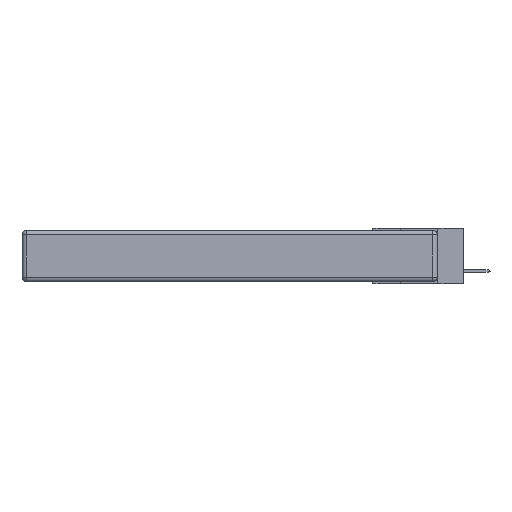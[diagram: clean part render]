
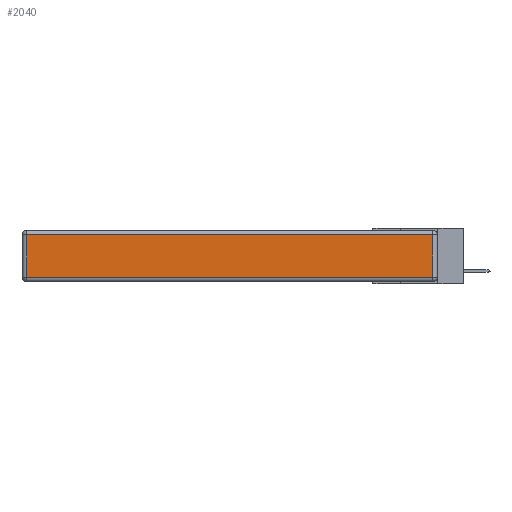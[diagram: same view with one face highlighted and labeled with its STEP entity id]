
A CAD part, left-side view. The second image highlights one B-rep face of the part: STEP entity #2040.
In plain terms, the highlighted planar face has unit normal (-1, 0, 0).
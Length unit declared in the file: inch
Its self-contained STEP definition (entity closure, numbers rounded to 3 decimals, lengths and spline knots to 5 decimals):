
#252 = VECTOR ( 'NONE', #1805, 39.37008 ) ;
#397 = CARTESIAN_POINT ( 'NONE',  ( 0., 2.72, -0.313 ) ) ;
#528 = CARTESIAN_POINT ( 'NONE',  ( 0., 0.03, -0.343 ) ) ;
#615 = EDGE_CURVE ( 'NONE', #8785, #6904, #5370, .T. ) ;
#1092 = ORIENTED_EDGE ( 'NONE', *, *, #615, .T. ) ;
#1435 = VECTOR ( 'NONE', #5784, 39.37008 ) ;
#1805 = DIRECTION ( 'NONE',  ( 0., 0., 1. ) ) ;
#2040 = ADVANCED_FACE ( 'NONE', ( #12250 ), #4690, .T. ) ;
#2450 = VERTEX_POINT ( 'NONE', #397 ) ;
#3896 = VECTOR ( 'NONE', #12464, 39.37008 ) ;
#4378 = EDGE_LOOP ( 'NONE', ( #11675, #1092, #7828, #9726 ) ) ;
#4491 = EDGE_CURVE ( 'NONE', #6904, #4691, #7237, .T. ) ;
#4690 = PLANE ( 'NONE',  #10611 ) ;
#4691 = VERTEX_POINT ( 'NONE', #9152 ) ;
#4716 = CARTESIAN_POINT ( 'NONE',  ( 0., 0.03, -0.313 ) ) ;
#4989 = LINE ( 'NONE', #13332, #1435 ) ;
#5370 = LINE ( 'NONE', #528, #252 ) ;
#5624 = CARTESIAN_POINT ( 'NONE',  ( 0., 0.03, -0.03 ) ) ;
#5784 = DIRECTION ( 'NONE',  ( 0., -1., 0. ) ) ;
#5982 = CARTESIAN_POINT ( 'NONE',  ( 0., 0., -0.343 ) ) ;
#6904 = VERTEX_POINT ( 'NONE', #5624 ) ;
#7237 = LINE ( 'NONE', #16169, #3896 ) ;
#7244 = DIRECTION ( 'NONE',  ( -1., 0., 0. ) ) ;
#7828 = ORIENTED_EDGE ( 'NONE', *, *, #4491, .T. ) ;
#8142 = EDGE_CURVE ( 'NONE', #2450, #8785, #4989, .T. ) ;
#8517 = DIRECTION ( 'NONE',  ( 0., 0., 1. ) ) ;
#8785 = VERTEX_POINT ( 'NONE', #4716 ) ;
#9152 = CARTESIAN_POINT ( 'NONE',  ( 0., 2.72, -0.03 ) ) ;
#9726 = ORIENTED_EDGE ( 'NONE', *, *, #14651, .T. ) ;
#10611 = AXIS2_PLACEMENT_3D ( 'NONE', #5982, #7244, #8517 ) ;
#11675 = ORIENTED_EDGE ( 'NONE', *, *, #8142, .T. ) ;
#12235 = VECTOR ( 'NONE', #15403, 39.37008 ) ;
#12250 = FACE_OUTER_BOUND ( 'NONE', #4378, .T. ) ;
#12464 = DIRECTION ( 'NONE',  ( 0., 1., 0. ) ) ;
#13018 = LINE ( 'NONE', #14205, #12235 ) ;
#13332 = CARTESIAN_POINT ( 'NONE',  ( 0., 0., -0.313 ) ) ;
#14205 = CARTESIAN_POINT ( 'NONE',  ( 0., 2.72, -0.343 ) ) ;
#14651 = EDGE_CURVE ( 'NONE', #4691, #2450, #13018, .T. ) ;
#15403 = DIRECTION ( 'NONE',  ( 0., 0., -1. ) ) ;
#16169 = CARTESIAN_POINT ( 'NONE',  ( 0., 2.75, -0.03 ) ) ;
